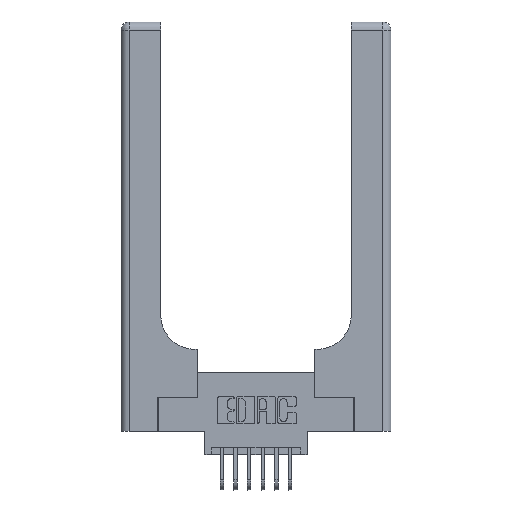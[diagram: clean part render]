
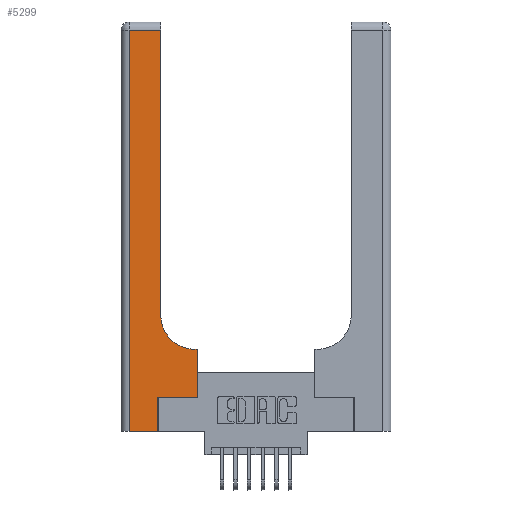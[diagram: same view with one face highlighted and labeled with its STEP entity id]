
A CAD part, top view. The second image highlights one B-rep face of the part: STEP entity #5299.
In plain terms, the highlighted planar face has unit normal (0, 0, 1).
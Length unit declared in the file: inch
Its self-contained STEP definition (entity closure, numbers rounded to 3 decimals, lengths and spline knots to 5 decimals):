
#72 = CARTESIAN_POINT ( 'NONE',  ( 0.06, 2.94, 0.37 ) ) ;
#205 = VECTOR ( 'NONE', #7796, 39.37008 ) ;
#550 = ORIENTED_EDGE ( 'NONE', *, *, #7018, .T. ) ;
#581 = DIRECTION ( 'NONE',  ( 0., -1., 0. ) ) ;
#632 = FACE_OUTER_BOUND ( 'NONE', #13905, .T. ) ;
#776 = VERTEX_POINT ( 'NONE', #15256 ) ;
#1461 = CARTESIAN_POINT ( 'NONE',  ( 0., 0., 0.37 ) ) ;
#1486 = DIRECTION ( 'NONE',  ( 0., 1., 0. ) ) ;
#2316 = ORIENTED_EDGE ( 'NONE', *, *, #13369, .T. ) ;
#2376 = ORIENTED_EDGE ( 'NONE', *, *, #12972, .T. ) ;
#3415 = LINE ( 'NONE', #6686, #16449 ) ;
#3432 = VERTEX_POINT ( 'NONE', #14047 ) ;
#3609 = ORIENTED_EDGE ( 'NONE', *, *, #9925, .T. ) ;
#4030 = VERTEX_POINT ( 'NONE', #5287 ) ;
#4474 = VERTEX_POINT ( 'NONE', #16173 ) ;
#4590 = LINE ( 'NONE', #12511, #7512 ) ;
#5287 = CARTESIAN_POINT ( 'NONE',  ( 0.269, 0.25, 0.37 ) ) ;
#5299 = ADVANCED_FACE ( 'NONE', ( #632 ), #11628, .F. ) ;
#5308 = CARTESIAN_POINT ( 'NONE',  ( 0., 3., 0.37 ) ) ;
#5323 = EDGE_CURVE ( 'NONE', #15144, #776, #12096, .T. ) ;
#5567 = LINE ( 'NONE', #6587, #11947 ) ;
#5726 = ORIENTED_EDGE ( 'NONE', *, *, #13158, .T. ) ;
#5816 = CARTESIAN_POINT ( 'NONE',  ( 0.5415, 0.85, 0.37 ) ) ;
#5957 = VECTOR ( 'NONE', #13771, 39.37008 ) ;
#6129 = EDGE_CURVE ( 'NONE', #3432, #11653, #6479, .T. ) ;
#6156 = LINE ( 'NONE', #15847, #12138 ) ;
#6381 = CARTESIAN_POINT ( 'NONE',  ( 0.2915, 3., 0.37 ) ) ;
#6450 = VECTOR ( 'NONE', #12918, 39.37008 ) ;
#6479 = CIRCLE ( 'NONE', #12866, 0.25 ) ;
#6558 = DIRECTION ( 'NONE',  ( -1., 0., 0. ) ) ;
#6587 = CARTESIAN_POINT ( 'NONE',  ( 0.5585, 0.25, 0.37 ) ) ;
#6632 = AXIS2_PLACEMENT_3D ( 'NONE', #5308, #14159, #6558 ) ;
#6686 = CARTESIAN_POINT ( 'NONE',  ( 0., 2.94, 0.37 ) ) ;
#6820 = LINE ( 'NONE', #10294, #6450 ) ;
#6933 = CARTESIAN_POINT ( 'NONE',  ( 0.2915, 0.85, 0.37 ) ) ;
#7018 = EDGE_CURVE ( 'NONE', #11969, #3432, #6820, .T. ) ;
#7054 = DIRECTION ( 'NONE',  ( 1., 0., 0. ) ) ;
#7512 = VECTOR ( 'NONE', #13755, 39.37008 ) ;
#7665 = DIRECTION ( 'NONE',  ( 0., 1., 0. ) ) ;
#7796 = DIRECTION ( 'NONE',  ( 1., 0., 0. ) ) ;
#7930 = DIRECTION ( 'NONE',  ( -1., 0., 0. ) ) ;
#8323 = VERTEX_POINT ( 'NONE', #11964 ) ;
#8675 = CARTESIAN_POINT ( 'NONE',  ( 0.06, 0., 0.37 ) ) ;
#8919 = EDGE_CURVE ( 'NONE', #8323, #15823, #3415, .T. ) ;
#9265 = LINE ( 'NONE', #11211, #5957 ) ;
#9563 = ORIENTED_EDGE ( 'NONE', *, *, #6129, .T. ) ;
#9925 = EDGE_CURVE ( 'NONE', #776, #4030, #9265, .T. ) ;
#10259 = CARTESIAN_POINT ( 'NONE',  ( 0.5585, 0.6, 0.37 ) ) ;
#10294 = CARTESIAN_POINT ( 'NONE',  ( 0.2915, 0.6, 0.37 ) ) ;
#10520 = EDGE_CURVE ( 'NONE', #11653, #8323, #11505, .T. ) ;
#11090 = VECTOR ( 'NONE', #7665, 39.37008 ) ;
#11211 = CARTESIAN_POINT ( 'NONE',  ( 0.269, 0., 0.37 ) ) ;
#11505 = LINE ( 'NONE', #6381, #11090 ) ;
#11628 = PLANE ( 'NONE',  #6632 ) ;
#11653 = VERTEX_POINT ( 'NONE', #6933 ) ;
#11947 = VECTOR ( 'NONE', #1486, 39.37008 ) ;
#11964 = CARTESIAN_POINT ( 'NONE',  ( 0.2915, 2.94, 0.37 ) ) ;
#11969 = VERTEX_POINT ( 'NONE', #10259 ) ;
#12096 = LINE ( 'NONE', #1461, #205 ) ;
#12138 = VECTOR ( 'NONE', #581, 39.37008 ) ;
#12511 = CARTESIAN_POINT ( 'NONE',  ( 0.269, 0.25, 0.37 ) ) ;
#12866 = AXIS2_PLACEMENT_3D ( 'NONE', #5816, #14653, #7054 ) ;
#12918 = DIRECTION ( 'NONE',  ( -1., 0., 0. ) ) ;
#12972 = EDGE_CURVE ( 'NONE', #4030, #4474, #4590, .T. ) ;
#13158 = EDGE_CURVE ( 'NONE', #4474, #11969, #5567, .T. ) ;
#13369 = EDGE_CURVE ( 'NONE', #15823, #15144, #6156, .T. ) ;
#13619 = ORIENTED_EDGE ( 'NONE', *, *, #5323, .T. ) ;
#13755 = DIRECTION ( 'NONE',  ( 1., 0., 0. ) ) ;
#13771 = DIRECTION ( 'NONE',  ( 0., 1., 0. ) ) ;
#13905 = EDGE_LOOP ( 'NONE', ( #14710, #16022, #2316, #13619, #3609, #2376, #5726, #550, #9563 ) ) ;
#14047 = CARTESIAN_POINT ( 'NONE',  ( 0.5415, 0.6, 0.37 ) ) ;
#14159 = DIRECTION ( 'NONE',  ( 0., 0., -1. ) ) ;
#14653 = DIRECTION ( 'NONE',  ( 0., 0., -1. ) ) ;
#14710 = ORIENTED_EDGE ( 'NONE', *, *, #10520, .T. ) ;
#15144 = VERTEX_POINT ( 'NONE', #8675 ) ;
#15256 = CARTESIAN_POINT ( 'NONE',  ( 0.269, 0., 0.37 ) ) ;
#15823 = VERTEX_POINT ( 'NONE', #72 ) ;
#15847 = CARTESIAN_POINT ( 'NONE',  ( 0.06, 3., 0.37 ) ) ;
#16022 = ORIENTED_EDGE ( 'NONE', *, *, #8919, .T. ) ;
#16173 = CARTESIAN_POINT ( 'NONE',  ( 0.5585, 0.25, 0.37 ) ) ;
#16449 = VECTOR ( 'NONE', #7930, 39.37008 ) ;
